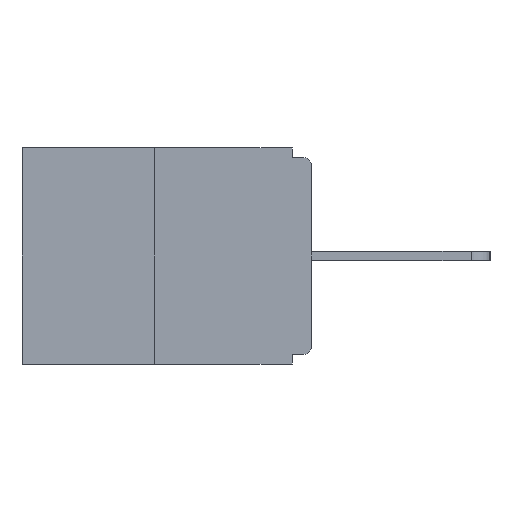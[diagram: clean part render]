
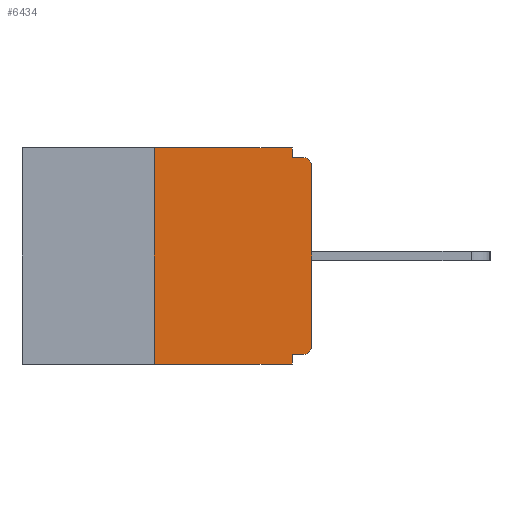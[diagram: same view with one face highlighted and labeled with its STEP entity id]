
A CAD part, left-side view. The second image highlights one B-rep face of the part: STEP entity #6434.
In plain terms, the highlighted planar face has unit normal (-1, 0, 0).
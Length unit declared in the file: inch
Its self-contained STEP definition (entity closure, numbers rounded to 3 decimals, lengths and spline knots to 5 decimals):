
#86 = VECTOR ( 'NONE', #9535, 39.37008 ) ;
#243 = AXIS2_PLACEMENT_3D ( 'NONE', #1606, #15671, #11319 ) ;
#567 = FACE_OUTER_BOUND ( 'NONE', #11091, .T. ) ;
#736 = ORIENTED_EDGE ( 'NONE', *, *, #15181, .F. ) ;
#807 = ORIENTED_EDGE ( 'NONE', *, *, #8666, .T. ) ;
#812 = LINE ( 'NONE', #10660, #7127 ) ;
#941 = ORIENTED_EDGE ( 'NONE', *, *, #8455, .F. ) ;
#1088 = ORIENTED_EDGE ( 'NONE', *, *, #7931, .T. ) ;
#1296 = DIRECTION ( 'NONE',  ( 0., -1., 0. ) ) ;
#1369 = EDGE_CURVE ( 'NONE', #14781, #4501, #8948, .T. ) ;
#1606 = CARTESIAN_POINT ( 'NONE',  ( 0., 0.015, -0.313 ) ) ;
#1992 = DIRECTION ( 'NONE',  ( 0., 1., 0. ) ) ;
#2161 = EDGE_CURVE ( 'NONE', #7897, #16139, #12150, .T. ) ;
#2490 = DIRECTION ( 'NONE',  ( 0., 0., -1. ) ) ;
#2580 = CARTESIAN_POINT ( 'NONE',  ( 0., 0.031, -0.343 ) ) ;
#2711 = CIRCLE ( 'NONE', #243, 0.015 ) ;
#2859 = VECTOR ( 'NONE', #7598, 39.37008 ) ;
#2867 = CARTESIAN_POINT ( 'NONE',  ( 0., 0.25, 0. ) ) ;
#3276 = DIRECTION ( 'NONE',  ( 0., -1., 0. ) ) ;
#3647 = VECTOR ( 'NONE', #8120, 39.37008 ) ;
#3739 = AXIS2_PLACEMENT_3D ( 'NONE', #14988, #16387, #15059 ) ;
#3891 = EDGE_CURVE ( 'NONE', #14173, #14781, #9453, .T. ) ;
#3898 = PLANE ( 'NONE',  #3739 ) ;
#4009 = VECTOR ( 'NONE', #3276, 39.37008 ) ;
#4266 = EDGE_CURVE ( 'NONE', #16139, #4501, #4430, .T. ) ;
#4430 = CIRCLE ( 'NONE', #6742, 0.015 ) ;
#4501 = VERTEX_POINT ( 'NONE', #11718 ) ;
#5027 = CARTESIAN_POINT ( 'NONE',  ( 0., 0.015, -0.03 ) ) ;
#5524 = LINE ( 'NONE', #17850, #12067 ) ;
#6434 = ADVANCED_FACE ( 'NONE', ( #567 ), #3898, .F. ) ;
#6742 = AXIS2_PLACEMENT_3D ( 'NONE', #5027, #12051, #7869 ) ;
#6769 = DIRECTION ( 'NONE',  ( 0., 0., 1. ) ) ;
#7127 = VECTOR ( 'NONE', #6769, 39.37008 ) ;
#7198 = VERTEX_POINT ( 'NONE', #13633 ) ;
#7394 = VERTEX_POINT ( 'NONE', #14709 ) ;
#7439 = CARTESIAN_POINT ( 'NONE',  ( 0., 0.031, -0.015 ) ) ;
#7598 = DIRECTION ( 'NONE',  ( 0., -1., 0. ) ) ;
#7646 = CARTESIAN_POINT ( 'NONE',  ( 0., 0., -0.328 ) ) ;
#7869 = DIRECTION ( 'NONE',  ( 0., 0., -1. ) ) ;
#7897 = VERTEX_POINT ( 'NONE', #17976 ) ;
#7931 = EDGE_CURVE ( 'NONE', #7394, #7897, #2711, .T. ) ;
#7970 = ORIENTED_EDGE ( 'NONE', *, *, #2161, .T. ) ;
#8120 = DIRECTION ( 'NONE',  ( 0., 0., 1. ) ) ;
#8455 = EDGE_CURVE ( 'NONE', #13919, #14173, #10983, .T. ) ;
#8570 = LINE ( 'NONE', #2580, #86 ) ;
#8619 = EDGE_CURVE ( 'NONE', #7198, #18034, #8570, .T. ) ;
#8630 = LINE ( 'NONE', #7646, #11471 ) ;
#8666 = EDGE_CURVE ( 'NONE', #13931, #18034, #5524, .T. ) ;
#8948 = LINE ( 'NONE', #15970, #2859 ) ;
#9453 = LINE ( 'NONE', #10304, #13342 ) ;
#9535 = DIRECTION ( 'NONE',  ( 0., 0., -1. ) ) ;
#9754 = CARTESIAN_POINT ( 'NONE',  ( 0., 0.25, -0.343 ) ) ;
#10304 = CARTESIAN_POINT ( 'NONE',  ( 0., 0.031, 0. ) ) ;
#10660 = CARTESIAN_POINT ( 'NONE',  ( 0., 0.25, 0. ) ) ;
#10983 = LINE ( 'NONE', #17147, #4009 ) ;
#11091 = EDGE_LOOP ( 'NONE', ( #941, #14118, #807, #13659, #736, #1088, #7970, #11513, #17303, #13865 ) ) ;
#11319 = DIRECTION ( 'NONE',  ( 0., 0., -1. ) ) ;
#11471 = VECTOR ( 'NONE', #1992, 39.37008 ) ;
#11513 = ORIENTED_EDGE ( 'NONE', *, *, #4266, .T. ) ;
#11718 = CARTESIAN_POINT ( 'NONE',  ( 0., 0.015, -0.015 ) ) ;
#12051 = DIRECTION ( 'NONE',  ( -1., 0., 0. ) ) ;
#12067 = VECTOR ( 'NONE', #1296, 39.37008 ) ;
#12150 = LINE ( 'NONE', #17737, #3647 ) ;
#12461 = CARTESIAN_POINT ( 'NONE',  ( 0., 0.031, 0. ) ) ;
#13342 = VECTOR ( 'NONE', #2490, 39.37008 ) ;
#13633 = CARTESIAN_POINT ( 'NONE',  ( 0., 0.031, -0.328 ) ) ;
#13659 = ORIENTED_EDGE ( 'NONE', *, *, #8619, .F. ) ;
#13865 = ORIENTED_EDGE ( 'NONE', *, *, #3891, .F. ) ;
#13919 = VERTEX_POINT ( 'NONE', #2867 ) ;
#13931 = VERTEX_POINT ( 'NONE', #9754 ) ;
#14118 = ORIENTED_EDGE ( 'NONE', *, *, #14384, .F. ) ;
#14173 = VERTEX_POINT ( 'NONE', #12461 ) ;
#14367 = CARTESIAN_POINT ( 'NONE',  ( 0., 0., -0.03 ) ) ;
#14384 = EDGE_CURVE ( 'NONE', #13931, #13919, #812, .T. ) ;
#14709 = CARTESIAN_POINT ( 'NONE',  ( 0., 0.015, -0.328 ) ) ;
#14781 = VERTEX_POINT ( 'NONE', #7439 ) ;
#14988 = CARTESIAN_POINT ( 'NONE',  ( 0., 0.46, 0. ) ) ;
#15059 = DIRECTION ( 'NONE',  ( 0., 0., -1. ) ) ;
#15181 = EDGE_CURVE ( 'NONE', #7394, #7198, #8630, .T. ) ;
#15469 = CARTESIAN_POINT ( 'NONE',  ( 0., 0.031, -0.343 ) ) ;
#15671 = DIRECTION ( 'NONE',  ( -1., 0., 0. ) ) ;
#15970 = CARTESIAN_POINT ( 'NONE',  ( 0., 0., -0.015 ) ) ;
#16139 = VERTEX_POINT ( 'NONE', #14367 ) ;
#16387 = DIRECTION ( 'NONE',  ( 1., 0., 0. ) ) ;
#17147 = CARTESIAN_POINT ( 'NONE',  ( 0., 0.46, 0. ) ) ;
#17303 = ORIENTED_EDGE ( 'NONE', *, *, #1369, .F. ) ;
#17737 = CARTESIAN_POINT ( 'NONE',  ( 0., 0., 0. ) ) ;
#17850 = CARTESIAN_POINT ( 'NONE',  ( 0., 0.46, -0.343 ) ) ;
#17976 = CARTESIAN_POINT ( 'NONE',  ( 0., 0., -0.313 ) ) ;
#18034 = VERTEX_POINT ( 'NONE', #15469 ) ;
